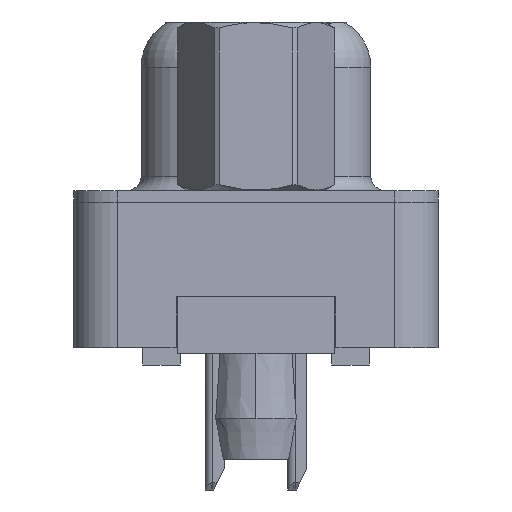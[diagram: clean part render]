
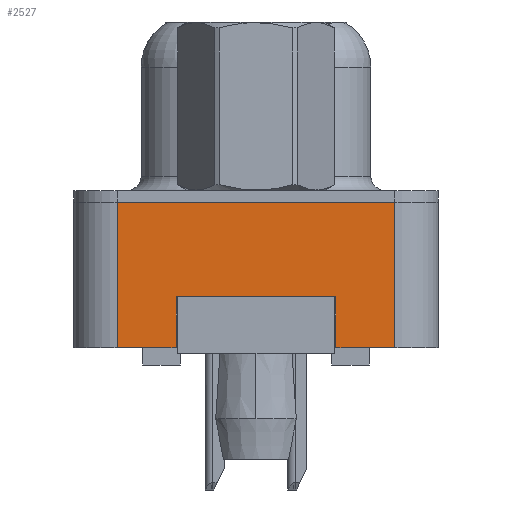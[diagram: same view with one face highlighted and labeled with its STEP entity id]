
A CAD part, left-side view. The second image highlights one B-rep face of the part: STEP entity #2527.
In plain terms, the highlighted planar face has unit normal (-1, 0, 0).
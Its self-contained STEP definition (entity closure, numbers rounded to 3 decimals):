
#521 = DIRECTION ( 'NONE',  ( -1., 0., 0. ) ) ;
#1189 = EDGE_CURVE ( 'NONE', #7157, #11529, #19105, .T. ) ;
#1598 = VERTEX_POINT ( 'NONE', #3487 ) ;
#1728 = ORIENTED_EDGE ( 'NONE', *, *, #3574, .T. ) ;
#1739 = CARTESIAN_POINT ( 'NONE',  ( -2.995, 2.75, -3.25 ) ) ;
#2527 = ADVANCED_FACE ( 'NONE', ( #6474 ), #9963, .T. ) ;
#3052 = VECTOR ( 'NONE', #10660, 1000. ) ;
#3064 = CARTESIAN_POINT ( 'NONE',  ( -2.995, -4.775, -5. ) ) ;
#3103 = EDGE_CURVE ( 'NONE', #1598, #11529, #13564, .T. ) ;
#3342 = CARTESIAN_POINT ( 'NONE',  ( -2.995, -2.75, -3.25 ) ) ;
#3487 = CARTESIAN_POINT ( 'NONE',  ( -2.995, 4.775, -5. ) ) ;
#3574 = EDGE_CURVE ( 'NONE', #15258, #21568, #10277, .T. ) ;
#3902 = CARTESIAN_POINT ( 'NONE',  ( -2.995, -4.775, -5. ) ) ;
#4069 = LINE ( 'NONE', #23042, #15082 ) ;
#4222 = CARTESIAN_POINT ( 'NONE',  ( -2.995, 4.775, -5. ) ) ;
#4527 = VECTOR ( 'NONE', #12740, 1000. ) ;
#4743 = EDGE_CURVE ( 'NONE', #21622, #7157, #4766, .T. ) ;
#4766 = LINE ( 'NONE', #12492, #4527 ) ;
#5118 = VECTOR ( 'NONE', #20959, 1000. ) ;
#6346 = LINE ( 'NONE', #4222, #21303 ) ;
#6474 = FACE_OUTER_BOUND ( 'NONE', #21105, .T. ) ;
#6587 = CARTESIAN_POINT ( 'NONE',  ( -2.995, 2.75, -5. ) ) ;
#7157 = VERTEX_POINT ( 'NONE', #1739 ) ;
#7935 = CARTESIAN_POINT ( 'NONE',  ( -2.995, -2.75, -3.25 ) ) ;
#8020 = EDGE_CURVE ( 'NONE', #21622, #11519, #9057, .T. ) ;
#8090 = DIRECTION ( 'NONE',  ( 0., 0., 1. ) ) ;
#8251 = ORIENTED_EDGE ( 'NONE', *, *, #21123, .F. ) ;
#8566 = ORIENTED_EDGE ( 'NONE', *, *, #1189, .F. ) ;
#8853 = ORIENTED_EDGE ( 'NONE', *, *, #9705, .T. ) ;
#9057 = LINE ( 'NONE', #3342, #22976 ) ;
#9705 = EDGE_CURVE ( 'NONE', #11519, #15258, #12539, .T. ) ;
#9810 = DIRECTION ( 'NONE',  ( 0., -1., 0. ) ) ;
#9963 = PLANE ( 'NONE',  #21509 ) ;
#10277 = LINE ( 'NONE', #12529, #23220 ) ;
#10344 = CARTESIAN_POINT ( 'NONE',  ( -2.995, -4.775, -5. ) ) ;
#10660 = DIRECTION ( 'NONE',  ( 0., -1., 0. ) ) ;
#11157 = ORIENTED_EDGE ( 'NONE', *, *, #4743, .F. ) ;
#11519 = VERTEX_POINT ( 'NONE', #16344 ) ;
#11529 = VERTEX_POINT ( 'NONE', #6587 ) ;
#11663 = DIRECTION ( 'NONE',  ( 0., -1., 0. ) ) ;
#11696 = DIRECTION ( 'NONE',  ( 0., 0., 1. ) ) ;
#12072 = EDGE_CURVE ( 'NONE', #21549, #21568, #4069, .T. ) ;
#12193 = VECTOR ( 'NONE', #9810, 1000. ) ;
#12492 = CARTESIAN_POINT ( 'NONE',  ( -2.995, 2.75, -3.25 ) ) ;
#12529 = CARTESIAN_POINT ( 'NONE',  ( -2.995, -4.775, -5. ) ) ;
#12539 = LINE ( 'NONE', #3064, #3052 ) ;
#12740 = DIRECTION ( 'NONE',  ( 0., 1., 0. ) ) ;
#13564 = LINE ( 'NONE', #19320, #12193 ) ;
#15082 = VECTOR ( 'NONE', #11663, 1000. ) ;
#15258 = VERTEX_POINT ( 'NONE', #3902 ) ;
#15350 = CARTESIAN_POINT ( 'NONE',  ( -2.995, 2.75, -3.25 ) ) ;
#16344 = CARTESIAN_POINT ( 'NONE',  ( -2.995, -2.75, -5. ) ) ;
#17073 = CARTESIAN_POINT ( 'NONE',  ( -2.995, -4.775, 0. ) ) ;
#18446 = ORIENTED_EDGE ( 'NONE', *, *, #12072, .F. ) ;
#19105 = LINE ( 'NONE', #15350, #5118 ) ;
#19320 = CARTESIAN_POINT ( 'NONE',  ( -2.995, -4.775, -5. ) ) ;
#20032 = DIRECTION ( 'NONE',  ( 0., 0., 1. ) ) ;
#20791 = DIRECTION ( 'NONE',  ( 0., 0., -1. ) ) ;
#20959 = DIRECTION ( 'NONE',  ( 0., 0., -1. ) ) ;
#20998 = ORIENTED_EDGE ( 'NONE', *, *, #8020, .T. ) ;
#21105 = EDGE_LOOP ( 'NONE', ( #20998, #8853, #1728, #18446, #8251, #22900, #8566, #11157 ) ) ;
#21123 = EDGE_CURVE ( 'NONE', #1598, #21549, #6346, .T. ) ;
#21303 = VECTOR ( 'NONE', #11696, 1000. ) ;
#21509 = AXIS2_PLACEMENT_3D ( 'NONE', #10344, #521, #8090 ) ;
#21549 = VERTEX_POINT ( 'NONE', #24312 ) ;
#21568 = VERTEX_POINT ( 'NONE', #17073 ) ;
#21622 = VERTEX_POINT ( 'NONE', #7935 ) ;
#22900 = ORIENTED_EDGE ( 'NONE', *, *, #3103, .T. ) ;
#22976 = VECTOR ( 'NONE', #20791, 1000. ) ;
#23042 = CARTESIAN_POINT ( 'NONE',  ( -2.995, -4.775, 0. ) ) ;
#23220 = VECTOR ( 'NONE', #20032, 1000. ) ;
#24312 = CARTESIAN_POINT ( 'NONE',  ( -2.995, 4.775, 0. ) ) ;
